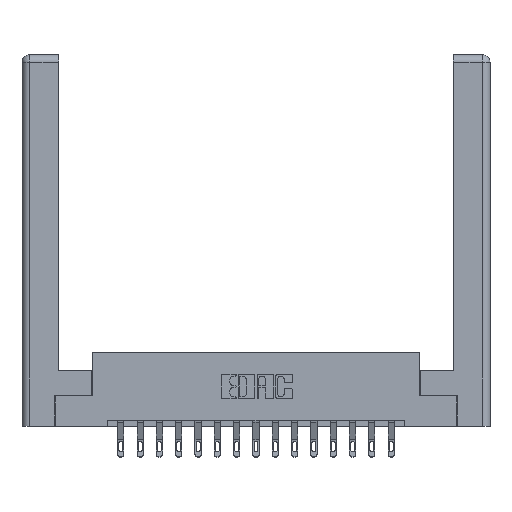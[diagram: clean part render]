
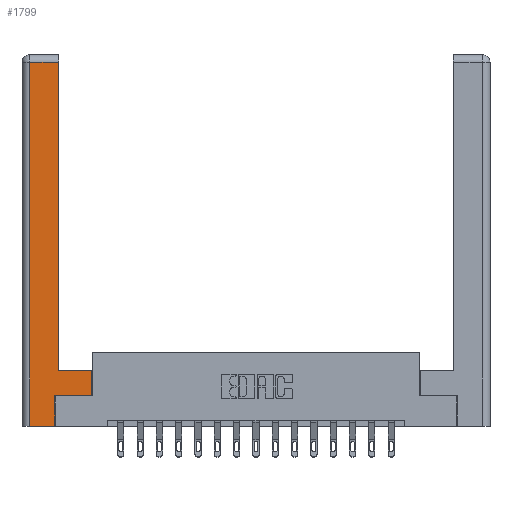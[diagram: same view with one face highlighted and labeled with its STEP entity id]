
A CAD part, top view. The second image highlights one B-rep face of the part: STEP entity #1799.
In plain terms, the highlighted planar face has unit normal (0, 0, 1).
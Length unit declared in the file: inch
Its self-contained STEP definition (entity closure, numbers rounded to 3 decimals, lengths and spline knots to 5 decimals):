
#457 = CARTESIAN_POINT ( 'NONE',  ( 0.0615, 2.94, 0. ) ) ;
#585 = CARTESIAN_POINT ( 'NONE',  ( 0.565, 0.245, 0. ) ) ;
#1054 = VECTOR ( 'NONE', #11440, 39.37008 ) ;
#1279 = LINE ( 'NONE', #15706, #3481 ) ;
#1336 = EDGE_CURVE ( 'NONE', #13288, #5557, #3500, .T. ) ;
#1799 = ADVANCED_FACE ( 'NONE', ( #2578 ), #5492, .F. ) ;
#1959 = DIRECTION ( 'NONE',  ( 1., 0., 0. ) ) ;
#2004 = EDGE_CURVE ( 'NONE', #5157, #3659, #14611, .T. ) ;
#2206 = VERTEX_POINT ( 'NONE', #7131 ) ;
#2223 = VERTEX_POINT ( 'NONE', #14224 ) ;
#2578 = FACE_OUTER_BOUND ( 'NONE', #9940, .T. ) ;
#2936 = CARTESIAN_POINT ( 'NONE',  ( 0.0615, 2.94, 0. ) ) ;
#3079 = LINE ( 'NONE', #585, #11356 ) ;
#3136 = EDGE_CURVE ( 'NONE', #5557, #5157, #13461, .T. ) ;
#3472 = EDGE_CURVE ( 'NONE', #12870, #2206, #12559, .T. ) ;
#3481 = VECTOR ( 'NONE', #17196, 39.37008 ) ;
#3500 = LINE ( 'NONE', #2936, #15721 ) ;
#3659 = VERTEX_POINT ( 'NONE', #7031 ) ;
#3827 = VECTOR ( 'NONE', #17953, 39.37008 ) ;
#3903 = AXIS2_PLACEMENT_3D ( 'NONE', #13658, #16558, #9544 ) ;
#4481 = EDGE_CURVE ( 'NONE', #13983, #2223, #3079, .T. ) ;
#4749 = VECTOR ( 'NONE', #14788, 39.37008 ) ;
#4904 = CARTESIAN_POINT ( 'NONE',  ( 0.0615, 0., 0. ) ) ;
#5009 = CARTESIAN_POINT ( 'NONE',  ( 0.295, 3., 0. ) ) ;
#5110 = ORIENTED_EDGE ( 'NONE', *, *, #4481, .T. ) ;
#5157 = VERTEX_POINT ( 'NONE', #16857 ) ;
#5272 = ORIENTED_EDGE ( 'NONE', *, *, #3472, .T. ) ;
#5492 = PLANE ( 'NONE',  #3903 ) ;
#5536 = ORIENTED_EDGE ( 'NONE', *, *, #15660, .T. ) ;
#5557 = VERTEX_POINT ( 'NONE', #457 ) ;
#5650 = EDGE_CURVE ( 'NONE', #2223, #12870, #1279, .T. ) ;
#5812 = CARTESIAN_POINT ( 'NONE',  ( 0.265, 0.245, 0. ) ) ;
#7031 = CARTESIAN_POINT ( 'NONE',  ( 0.265, 0., 0. ) ) ;
#7131 = CARTESIAN_POINT ( 'NONE',  ( 0.295, 0.45, 0. ) ) ;
#7640 = ORIENTED_EDGE ( 'NONE', *, *, #1336, .T. ) ;
#8698 = CARTESIAN_POINT ( 'NONE',  ( 0.265, 0., 0. ) ) ;
#9333 = CARTESIAN_POINT ( 'NONE',  ( 0.295, 0.45, 0. ) ) ;
#9437 = CARTESIAN_POINT ( 'NONE',  ( 0.295, 2.94, 0. ) ) ;
#9499 = ORIENTED_EDGE ( 'NONE', *, *, #14545, .T. ) ;
#9544 = DIRECTION ( 'NONE',  ( -1., 0., 0. ) ) ;
#9940 = EDGE_LOOP ( 'NONE', ( #9499, #7640, #17812, #13594, #5536, #5110, #12246, #5272 ) ) ;
#11356 = VECTOR ( 'NONE', #1959, 39.37008 ) ;
#11440 = DIRECTION ( 'NONE',  ( 1., 0., 0. ) ) ;
#11531 = DIRECTION ( 'NONE',  ( 0., 1., 0. ) ) ;
#12246 = ORIENTED_EDGE ( 'NONE', *, *, #5650, .T. ) ;
#12559 = LINE ( 'NONE', #9333, #3827 ) ;
#12870 = VERTEX_POINT ( 'NONE', #17442 ) ;
#12967 = CARTESIAN_POINT ( 'NONE',  ( 0.265, 0.245, 0. ) ) ;
#13237 = VECTOR ( 'NONE', #17507, 39.37008 ) ;
#13288 = VERTEX_POINT ( 'NONE', #9437 ) ;
#13461 = LINE ( 'NONE', #4904, #13237 ) ;
#13594 = ORIENTED_EDGE ( 'NONE', *, *, #2004, .T. ) ;
#13658 = CARTESIAN_POINT ( 'NONE',  ( 0., 0., 0. ) ) ;
#13983 = VERTEX_POINT ( 'NONE', #12967 ) ;
#14224 = CARTESIAN_POINT ( 'NONE',  ( 0.565, 0.245, 0. ) ) ;
#14362 = LINE ( 'NONE', #5009, #4749 ) ;
#14545 = EDGE_CURVE ( 'NONE', #2206, #13288, #14362, .T. ) ;
#14611 = LINE ( 'NONE', #8698, #1054 ) ;
#14788 = DIRECTION ( 'NONE',  ( 0., 1., 0. ) ) ;
#15223 = DIRECTION ( 'NONE',  ( -1., 0., 0. ) ) ;
#15618 = LINE ( 'NONE', #5812, #16960 ) ;
#15660 = EDGE_CURVE ( 'NONE', #3659, #13983, #15618, .T. ) ;
#15706 = CARTESIAN_POINT ( 'NONE',  ( 0.565, 0.45, 0. ) ) ;
#15721 = VECTOR ( 'NONE', #15223, 39.37008 ) ;
#16558 = DIRECTION ( 'NONE',  ( 0., 0., -1. ) ) ;
#16857 = CARTESIAN_POINT ( 'NONE',  ( 0.0615, 0., 0. ) ) ;
#16960 = VECTOR ( 'NONE', #11531, 39.37008 ) ;
#17196 = DIRECTION ( 'NONE',  ( 0., 1., 0. ) ) ;
#17442 = CARTESIAN_POINT ( 'NONE',  ( 0.565, 0.45, 0. ) ) ;
#17507 = DIRECTION ( 'NONE',  ( 0., -1., 0. ) ) ;
#17812 = ORIENTED_EDGE ( 'NONE', *, *, #3136, .T. ) ;
#17953 = DIRECTION ( 'NONE',  ( -1., 0., 0. ) ) ;
